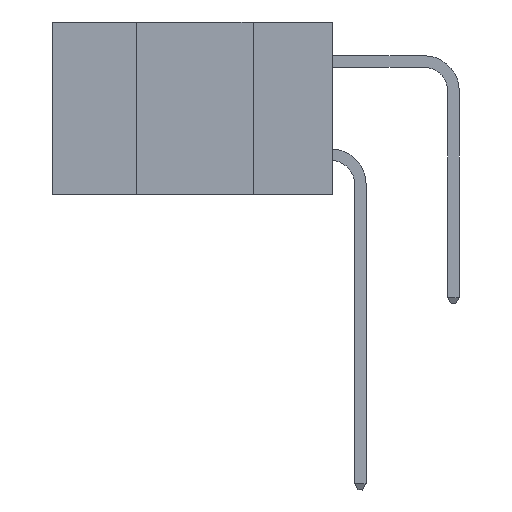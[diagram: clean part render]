
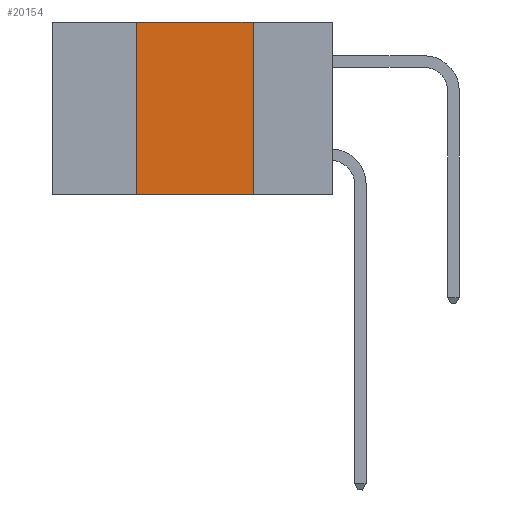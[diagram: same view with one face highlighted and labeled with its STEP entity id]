
A CAD part, left-side view. The second image highlights one B-rep face of the part: STEP entity #20154.
In plain terms, the highlighted planar face has unit normal (-1, 0, 0).
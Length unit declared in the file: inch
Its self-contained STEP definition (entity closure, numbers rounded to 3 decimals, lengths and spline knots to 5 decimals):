
#16 = VECTOR ( 'NONE', #201, 39.37008 ) ;
#201 = DIRECTION ( 'NONE',  ( 0., 0., 1. ) ) ;
#1160 = LINE ( 'NONE', #16954, #20825 ) ;
#1542 = CARTESIAN_POINT ( 'NONE',  ( 0., 0.42, -0.37 ) ) ;
#1811 = CARTESIAN_POINT ( 'NONE',  ( 0., 0.42, -0.37 ) ) ;
#2255 = VECTOR ( 'NONE', #18115, 39.37008 ) ;
#2881 = LINE ( 'NONE', #13059, #6159 ) ;
#3323 = PLANE ( 'NONE',  #21541 ) ;
#4188 = ORIENTED_EDGE ( 'NONE', *, *, #18048, .F. ) ;
#4756 = VERTEX_POINT ( 'NONE', #1542 ) ;
#4950 = DIRECTION ( 'NONE',  ( 0., 0., -1. ) ) ;
#6159 = VECTOR ( 'NONE', #20076, 39.37008 ) ;
#6265 = VERTEX_POINT ( 'NONE', #21282 ) ;
#6872 = CARTESIAN_POINT ( 'NONE',  ( 0., 0.17, 0. ) ) ;
#7429 = EDGE_CURVE ( 'NONE', #18023, #6265, #2881, .T. ) ;
#7627 = CARTESIAN_POINT ( 'NONE',  ( 0., 0.6, 0. ) ) ;
#8200 = DIRECTION ( 'NONE',  ( 0., -1., 0. ) ) ;
#8536 = DIRECTION ( 'NONE',  ( 1., 0., 0. ) ) ;
#9369 = ORIENTED_EDGE ( 'NONE', *, *, #21218, .T. ) ;
#11103 = LINE ( 'NONE', #7627, #2255 ) ;
#11707 = ORIENTED_EDGE ( 'NONE', *, *, #7429, .F. ) ;
#12167 = VERTEX_POINT ( 'NONE', #13269 ) ;
#13059 = CARTESIAN_POINT ( 'NONE',  ( 0., 0.17, -0.37 ) ) ;
#13269 = CARTESIAN_POINT ( 'NONE',  ( 0., 0.42, 0. ) ) ;
#13626 = FACE_OUTER_BOUND ( 'NONE', #18160, .T. ) ;
#16954 = CARTESIAN_POINT ( 'NONE',  ( 0., 0.6, -0.37 ) ) ;
#17402 = CARTESIAN_POINT ( 'NONE',  ( 0., 0.6, 0. ) ) ;
#18023 = VERTEX_POINT ( 'NONE', #6872 ) ;
#18048 = EDGE_CURVE ( 'NONE', #12167, #18023, #11103, .T. ) ;
#18115 = DIRECTION ( 'NONE',  ( 0., -1., 0. ) ) ;
#18160 = EDGE_LOOP ( 'NONE', ( #11707, #4188, #22675, #9369 ) ) ;
#18940 = EDGE_CURVE ( 'NONE', #4756, #12167, #21199, .T. ) ;
#20076 = DIRECTION ( 'NONE',  ( 0., 0., -1. ) ) ;
#20154 = ADVANCED_FACE ( 'NONE', ( #13626 ), #3323, .F. ) ;
#20825 = VECTOR ( 'NONE', #8200, 39.37008 ) ;
#21199 = LINE ( 'NONE', #1811, #16 ) ;
#21218 = EDGE_CURVE ( 'NONE', #4756, #6265, #1160, .T. ) ;
#21282 = CARTESIAN_POINT ( 'NONE',  ( 0., 0.17, -0.37 ) ) ;
#21541 = AXIS2_PLACEMENT_3D ( 'NONE', #17402, #8536, #4950 ) ;
#22675 = ORIENTED_EDGE ( 'NONE', *, *, #18940, .F. ) ;
